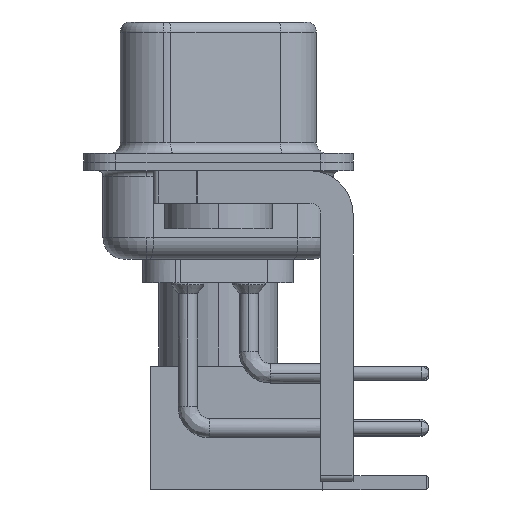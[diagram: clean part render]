
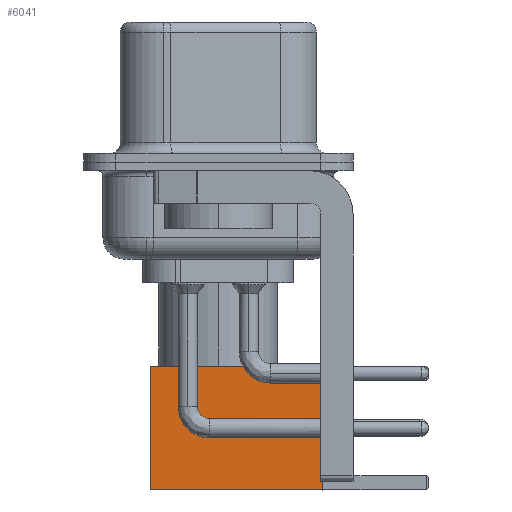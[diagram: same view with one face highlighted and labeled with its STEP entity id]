
A CAD part, left-side view. The second image highlights one B-rep face of the part: STEP entity #6041.
In plain terms, the highlighted face is planar.
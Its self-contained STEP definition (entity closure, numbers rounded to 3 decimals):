
#1112 = FACE_OUTER_BOUND ( 'NONE', #9468, .T. ) ;
#1216 = ORIENTED_EDGE ( 'NONE', *, *, #25567, .T. ) ;
#1508 = DIRECTION ( 'NONE',  ( 0., 0., -1. ) ) ;
#1643 = VERTEX_POINT ( 'NONE', #22414 ) ;
#2303 = CARTESIAN_POINT ( 'NONE',  ( 0., 2.875, 8. ) ) ;
#2427 = VECTOR ( 'NONE', #12233, 1000. ) ;
#2651 = ORIENTED_EDGE ( 'NONE', *, *, #3362, .F. ) ;
#3362 = EDGE_CURVE ( 'NONE', #15596, #19850, #20396, .T. ) ;
#3379 = CARTESIAN_POINT ( 'NONE',  ( -2.875, 2.875, 0. ) ) ;
#3850 = CARTESIAN_POINT ( 'NONE',  ( -2.875, 2.875, 8. ) ) ;
#4954 = CARTESIAN_POINT ( 'NONE',  ( 2.875, 2.875, 0. ) ) ;
#5224 = CARTESIAN_POINT ( 'NONE',  ( -2.875, 2.875, 0. ) ) ;
#5306 = ORIENTED_EDGE ( 'NONE', *, *, #19608, .T. ) ;
#5761 = CARTESIAN_POINT ( 'NONE',  ( 0., 2.875, 0. ) ) ;
#6041 = ADVANCED_FACE ( 'NONE', ( #1112 ), #23871, .T. ) ;
#6431 = LINE ( 'NONE', #2303, #20230 ) ;
#7993 = EDGE_CURVE ( 'NONE', #1643, #15596, #6431, .T. ) ;
#9468 = EDGE_LOOP ( 'NONE', ( #1216, #5306, #2651, #26755 ) ) ;
#10293 = LINE ( 'NONE', #5761, #2427 ) ;
#10554 = VECTOR ( 'NONE', #13547, 1000. ) ;
#10708 = DIRECTION ( 'NONE',  ( -1., 0., 0. ) ) ;
#12233 = DIRECTION ( 'NONE',  ( -1., 0., 0. ) ) ;
#13394 = DIRECTION ( 'NONE',  ( 0., 1., 0. ) ) ;
#13547 = DIRECTION ( 'NONE',  ( 0., 0., -1. ) ) ;
#15596 = VERTEX_POINT ( 'NONE', #3850 ) ;
#16292 = LINE ( 'NONE', #22359, #10554 ) ;
#19052 = VERTEX_POINT ( 'NONE', #25980 ) ;
#19608 = EDGE_CURVE ( 'NONE', #19052, #19850, #10293, .T. ) ;
#19850 = VERTEX_POINT ( 'NONE', #3379 ) ;
#20230 = VECTOR ( 'NONE', #10708, 1000. ) ;
#20396 = LINE ( 'NONE', #5224, #23222 ) ;
#21797 = DIRECTION ( 'NONE',  ( 0., 0., 1. ) ) ;
#22359 = CARTESIAN_POINT ( 'NONE',  ( 2.875, 2.875, 0. ) ) ;
#22414 = CARTESIAN_POINT ( 'NONE',  ( 2.875, 2.875, 8. ) ) ;
#23222 = VECTOR ( 'NONE', #1508, 1000. ) ;
#23871 = PLANE ( 'NONE',  #25578 ) ;
#25567 = EDGE_CURVE ( 'NONE', #1643, #19052, #16292, .T. ) ;
#25578 = AXIS2_PLACEMENT_3D ( 'NONE', #4954, #13394, #21797 ) ;
#25980 = CARTESIAN_POINT ( 'NONE',  ( 2.875, 2.875, 0. ) ) ;
#26755 = ORIENTED_EDGE ( 'NONE', *, *, #7993, .F. ) ;
